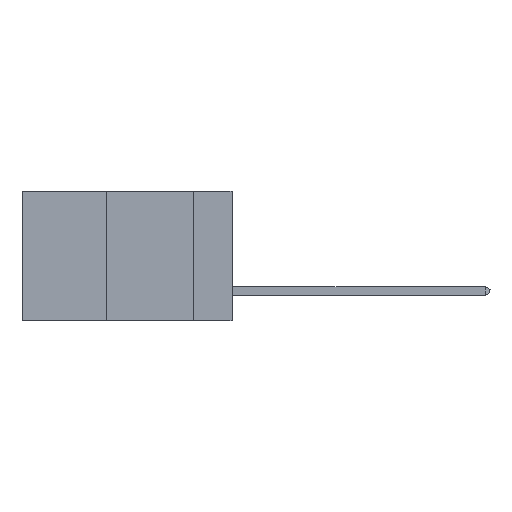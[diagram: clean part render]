
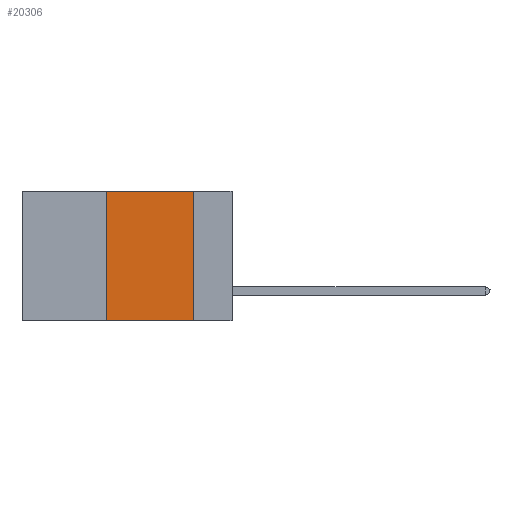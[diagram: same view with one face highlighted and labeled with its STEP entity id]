
A CAD part, left-side view. The second image highlights one B-rep face of the part: STEP entity #20306.
In plain terms, the highlighted planar face has unit normal (-1, 0, 0).
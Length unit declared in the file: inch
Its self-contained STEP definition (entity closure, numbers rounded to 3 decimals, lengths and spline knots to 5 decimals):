
#673 = CARTESIAN_POINT ( 'NONE',  ( 0., 0.6, 0. ) ) ;
#4467 = VECTOR ( 'NONE', #21120, 39.37008 ) ;
#7040 = VECTOR ( 'NONE', #44953, 39.37008 ) ;
#7515 = CARTESIAN_POINT ( 'NONE',  ( 0., 0.6, -0.37 ) ) ;
#10468 = VERTEX_POINT ( 'NONE', #36725 ) ;
#11545 = EDGE_CURVE ( 'NONE', #18981, #13942, #23760, .T. ) ;
#12308 = DIRECTION ( 'NONE',  ( 0., 0., -1. ) ) ;
#12569 = EDGE_CURVE ( 'NONE', #18981, #47222, #46264, .T. ) ;
#13040 = EDGE_LOOP ( 'NONE', ( #18233, #23172, #31651, #34434 ) ) ;
#13528 = LINE ( 'NONE', #13788, #7040 ) ;
#13788 = CARTESIAN_POINT ( 'NONE',  ( 0., 0.11, 0. ) ) ;
#13942 = VERTEX_POINT ( 'NONE', #16629 ) ;
#13975 = AXIS2_PLACEMENT_3D ( 'NONE', #673, #39318, #12308 ) ;
#16592 = LINE ( 'NONE', #47430, #35150 ) ;
#16629 = CARTESIAN_POINT ( 'NONE',  ( 0., 0.36, 0. ) ) ;
#18233 = ORIENTED_EDGE ( 'NONE', *, *, #38693, .F. ) ;
#18971 = EDGE_CURVE ( 'NONE', #13942, #10468, #16592, .T. ) ;
#18981 = VERTEX_POINT ( 'NONE', #28186 ) ;
#19823 = PLANE ( 'NONE',  #13975 ) ;
#20306 = ADVANCED_FACE ( 'NONE', ( #34955 ), #19823, .F. ) ;
#21120 = DIRECTION ( 'NONE',  ( 0., -1., 0. ) ) ;
#22297 = CARTESIAN_POINT ( 'NONE',  ( 0., 0.11, -0.37 ) ) ;
#23172 = ORIENTED_EDGE ( 'NONE', *, *, #18971, .F. ) ;
#23760 = LINE ( 'NONE', #43890, #41740 ) ;
#27834 = DIRECTION ( 'NONE',  ( 0., -1., 0. ) ) ;
#28186 = CARTESIAN_POINT ( 'NONE',  ( 0., 0.36, -0.37 ) ) ;
#31651 = ORIENTED_EDGE ( 'NONE', *, *, #11545, .F. ) ;
#32842 = DIRECTION ( 'NONE',  ( 0., 0., 1. ) ) ;
#34434 = ORIENTED_EDGE ( 'NONE', *, *, #12569, .T. ) ;
#34955 = FACE_OUTER_BOUND ( 'NONE', #13040, .T. ) ;
#35150 = VECTOR ( 'NONE', #27834, 39.37008 ) ;
#36725 = CARTESIAN_POINT ( 'NONE',  ( 0., 0.11, 0. ) ) ;
#38693 = EDGE_CURVE ( 'NONE', #10468, #47222, #13528, .T. ) ;
#39318 = DIRECTION ( 'NONE',  ( 1., 0., 0. ) ) ;
#41740 = VECTOR ( 'NONE', #32842, 39.37008 ) ;
#43890 = CARTESIAN_POINT ( 'NONE',  ( 0., 0.36, 0. ) ) ;
#44953 = DIRECTION ( 'NONE',  ( 0., 0., -1. ) ) ;
#46264 = LINE ( 'NONE', #7515, #4467 ) ;
#47222 = VERTEX_POINT ( 'NONE', #22297 ) ;
#47430 = CARTESIAN_POINT ( 'NONE',  ( 0., 0.6, 0. ) ) ;
